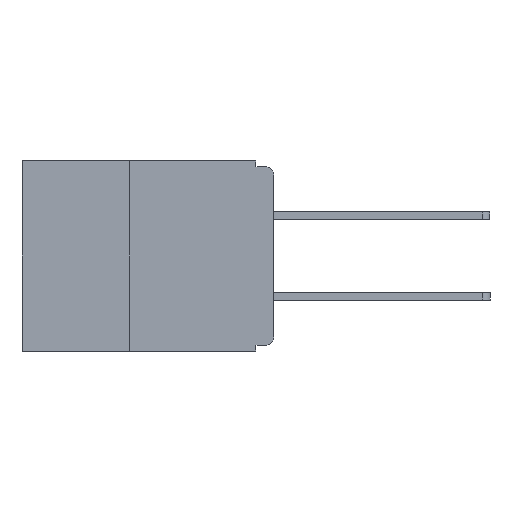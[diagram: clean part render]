
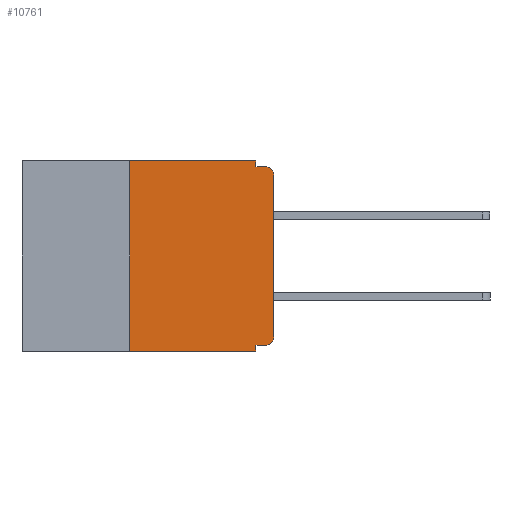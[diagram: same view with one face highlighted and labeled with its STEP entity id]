
A CAD part, left-side view. The second image highlights one B-rep face of the part: STEP entity #10761.
In plain terms, the highlighted planar face has unit normal (-1, 0, 0).
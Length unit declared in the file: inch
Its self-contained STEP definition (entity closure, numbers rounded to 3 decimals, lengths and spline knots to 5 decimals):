
#684 = VECTOR ( 'NONE', #22130, 39.37008 ) ;
#863 = LINE ( 'NONE', #10142, #4752 ) ;
#1021 = ORIENTED_EDGE ( 'NONE', *, *, #19514, .T. ) ;
#1150 = EDGE_CURVE ( 'NONE', #10254, #6626, #21584, .T. ) ;
#1323 = CARTESIAN_POINT ( 'NONE',  ( 0., 0.25, -0.33 ) ) ;
#1350 = ORIENTED_EDGE ( 'NONE', *, *, #8620, .T. ) ;
#1372 = ORIENTED_EDGE ( 'NONE', *, *, #2592, .F. ) ;
#1757 = LINE ( 'NONE', #5647, #5662 ) ;
#1782 = DIRECTION ( 'NONE',  ( 0., 0., -1. ) ) ;
#1998 = CARTESIAN_POINT ( 'NONE',  ( 0., 0.031, -0.01 ) ) ;
#2204 = CARTESIAN_POINT ( 'NONE',  ( 0., 0., -0.32 ) ) ;
#2217 = ORIENTED_EDGE ( 'NONE', *, *, #17690, .F. ) ;
#2437 = VERTEX_POINT ( 'NONE', #1998 ) ;
#2463 = ORIENTED_EDGE ( 'NONE', *, *, #9103, .F. ) ;
#2501 = DIRECTION ( 'NONE',  ( 0., 1., 0. ) ) ;
#2592 = EDGE_CURVE ( 'NONE', #2437, #19016, #10731, .T. ) ;
#2968 = CARTESIAN_POINT ( 'NONE',  ( 0., 0.437, 0. ) ) ;
#3129 = VECTOR ( 'NONE', #20119, 39.37008 ) ;
#3166 = VERTEX_POINT ( 'NONE', #23267 ) ;
#3346 = ORIENTED_EDGE ( 'NONE', *, *, #23909, .F. ) ;
#3515 = ORIENTED_EDGE ( 'NONE', *, *, #10902, .T. ) ;
#3923 = ORIENTED_EDGE ( 'NONE', *, *, #19289, .F. ) ;
#4125 = ORIENTED_EDGE ( 'NONE', *, *, #1150, .F. ) ;
#4237 = ORIENTED_EDGE ( 'NONE', *, *, #6028, .T. ) ;
#4301 = CARTESIAN_POINT ( 'NONE',  ( 0., 0.437, 0. ) ) ;
#4752 = VECTOR ( 'NONE', #15593, 39.37008 ) ;
#4905 = DIRECTION ( 'NONE',  ( 1., 0., 0. ) ) ;
#5426 = CARTESIAN_POINT ( 'NONE',  ( 0., 0.25, -0.33 ) ) ;
#5647 = CARTESIAN_POINT ( 'NONE',  ( 0., 0.031, -0.33 ) ) ;
#5662 = VECTOR ( 'NONE', #1782, 39.37008 ) ;
#5708 = VECTOR ( 'NONE', #16513, 39.37008 ) ;
#6028 = EDGE_CURVE ( 'NONE', #10254, #21668, #23209, .T. ) ;
#6092 = VERTEX_POINT ( 'NONE', #1323 ) ;
#6310 = LINE ( 'NONE', #16443, #5708 ) ;
#6626 = VERTEX_POINT ( 'NONE', #14141 ) ;
#6821 = DIRECTION ( 'NONE',  ( -1., 0., 0. ) ) ;
#7180 = DIRECTION ( 'NONE',  ( 0., -1., 0. ) ) ;
#8620 = EDGE_CURVE ( 'NONE', #21722, #19016, #14348, .T. ) ;
#8725 = LINE ( 'NONE', #5426, #3129 ) ;
#8760 = VECTOR ( 'NONE', #2501, 39.37008 ) ;
#9103 = EDGE_CURVE ( 'NONE', #16462, #3166, #13765, .T. ) ;
#9577 = VERTEX_POINT ( 'NONE', #13057 ) ;
#10142 = CARTESIAN_POINT ( 'NONE',  ( 0., 0., 0. ) ) ;
#10254 = VERTEX_POINT ( 'NONE', #16780 ) ;
#10616 = CARTESIAN_POINT ( 'NONE',  ( 0., 0.015, -0.025 ) ) ;
#10731 = LINE ( 'NONE', #20822, #684 ) ;
#10761 = ADVANCED_FACE ( 'NONE', ( #12154 ), #14143, .F. ) ;
#10889 = CARTESIAN_POINT ( 'NONE',  ( 0., 0.25, 0. ) ) ;
#10902 = EDGE_CURVE ( 'NONE', #6092, #9577, #18967, .T. ) ;
#11470 = CARTESIAN_POINT ( 'NONE',  ( 0., 0., -0.305 ) ) ;
#11868 = AXIS2_PLACEMENT_3D ( 'NONE', #10616, #23298, #12466 ) ;
#12154 = FACE_OUTER_BOUND ( 'NONE', #21939, .T. ) ;
#12466 = DIRECTION ( 'NONE',  ( 0., 0., -1. ) ) ;
#12709 = CARTESIAN_POINT ( 'NONE',  ( 0., 0.437, -0.33 ) ) ;
#12959 = CARTESIAN_POINT ( 'NONE',  ( 0., 0.015, -0.01 ) ) ;
#13057 = CARTESIAN_POINT ( 'NONE',  ( 0., 0.031, -0.33 ) ) ;
#13577 = VECTOR ( 'NONE', #7180, 39.37008 ) ;
#13765 = LINE ( 'NONE', #4301, #23371 ) ;
#14141 = CARTESIAN_POINT ( 'NONE',  ( 0., 0.031, -0.32 ) ) ;
#14143 = PLANE ( 'NONE',  #14766 ) ;
#14348 = CIRCLE ( 'NONE', #11868, 0.015 ) ;
#14766 = AXIS2_PLACEMENT_3D ( 'NONE', #2968, #4905, #17774 ) ;
#15593 = DIRECTION ( 'NONE',  ( 0., 0., 1. ) ) ;
#16443 = CARTESIAN_POINT ( 'NONE',  ( 0., 0.031, 0. ) ) ;
#16462 = VERTEX_POINT ( 'NONE', #10889 ) ;
#16513 = DIRECTION ( 'NONE',  ( 0., 0., -1. ) ) ;
#16780 = CARTESIAN_POINT ( 'NONE',  ( 0., 0.015, -0.32 ) ) ;
#17247 = DIRECTION ( 'NONE',  ( 0., -1., 0. ) ) ;
#17690 = EDGE_CURVE ( 'NONE', #3166, #2437, #6310, .T. ) ;
#17774 = DIRECTION ( 'NONE',  ( 0., 0., -1. ) ) ;
#17805 = CARTESIAN_POINT ( 'NONE',  ( 0., 0.015, -0.305 ) ) ;
#18049 = AXIS2_PLACEMENT_3D ( 'NONE', #17805, #6821, #19632 ) ;
#18967 = LINE ( 'NONE', #12709, #13577 ) ;
#19016 = VERTEX_POINT ( 'NONE', #12959 ) ;
#19289 = EDGE_CURVE ( 'NONE', #6626, #9577, #1757, .T. ) ;
#19514 = EDGE_CURVE ( 'NONE', #21668, #21722, #863, .T. ) ;
#19632 = DIRECTION ( 'NONE',  ( 0., 0., -1. ) ) ;
#20119 = DIRECTION ( 'NONE',  ( 0., 0., 1. ) ) ;
#20822 = CARTESIAN_POINT ( 'NONE',  ( 0., 0., -0.01 ) ) ;
#21584 = LINE ( 'NONE', #2204, #8760 ) ;
#21668 = VERTEX_POINT ( 'NONE', #11470 ) ;
#21722 = VERTEX_POINT ( 'NONE', #22403 ) ;
#21939 = EDGE_LOOP ( 'NONE', ( #1021, #1350, #1372, #2217, #2463, #3346, #3515, #3923, #4125, #4237 ) ) ;
#22130 = DIRECTION ( 'NONE',  ( 0., -1., 0. ) ) ;
#22403 = CARTESIAN_POINT ( 'NONE',  ( 0., 0., -0.025 ) ) ;
#23209 = CIRCLE ( 'NONE', #18049, 0.015 ) ;
#23267 = CARTESIAN_POINT ( 'NONE',  ( 0., 0.031, 0. ) ) ;
#23298 = DIRECTION ( 'NONE',  ( -1., 0., 0. ) ) ;
#23371 = VECTOR ( 'NONE', #17247, 39.37008 ) ;
#23909 = EDGE_CURVE ( 'NONE', #6092, #16462, #8725, .T. ) ;
